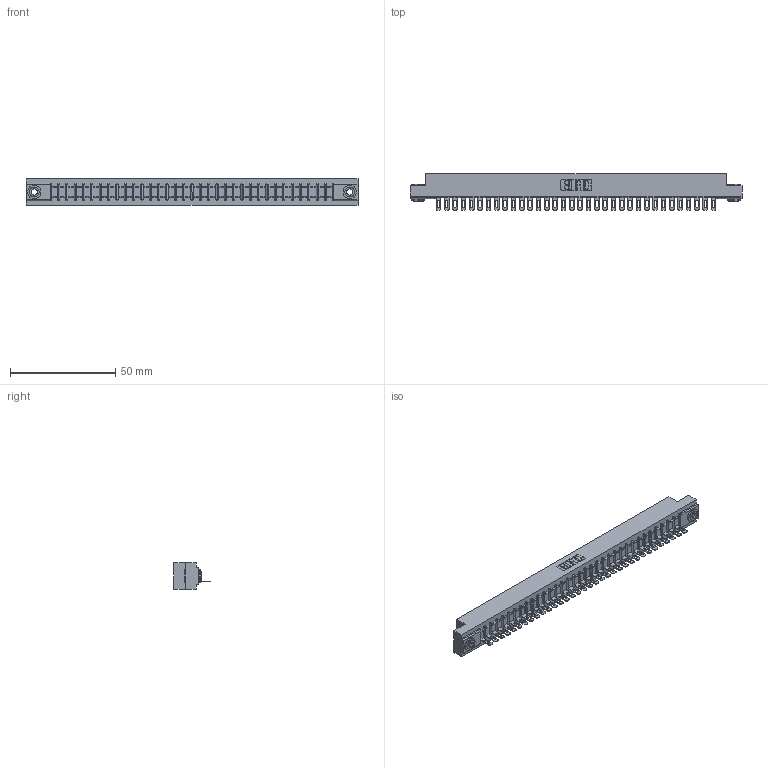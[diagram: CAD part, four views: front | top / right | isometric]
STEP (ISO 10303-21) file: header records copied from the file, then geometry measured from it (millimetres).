
FILE_DESCRIPTION (( 'STEP AP203' ), '1' );
FILE_NAME ('357-034-501-103.STEP', '2019-09-17T05:12:15', ( '' ), ( '' ), 'SwSTEP 2.0', 'SolidWorks 2016', '' );
FILE_SCHEMA (( 'CONFIG_CONTROL_DESIGN' ));
Length unit declared in the file: inch
Products named in the file (4): 307-290-002_501; 307 Part_.156 Dia Mounting Holes; 357-034-501-103; 345-250-002_345-250-002-102
Assembly tree (37 placements, depth 2):
  357-034-501-103
    307 Part_.156 Dia Mounting Holes
    307-290-002_501  x34
    345-250-002_345-250-002-102  x2
Bounding box: 157.73 x 17.42 x 12.7 mm (x, y, z)
Volume: 16850.8 mm3; surface area: 21491.2 mm2
Topology: 37 solids, 37 shells, 2789 faces, 8527 edges, 5586 vertices
Faces by surface type: plane 1590, cylinder 1121, sphere 70, cone 8
Entity records: 31993 total; most frequent: CARTESIAN_POINT 5373, ORIENTED_EDGE 5354, DIRECTION 5243, EDGE_CURVE 2677, LINE 2035, VECTOR 2035, VERTEX_POINT 1734, AXIS2_PLACEMENT_3D 1604
